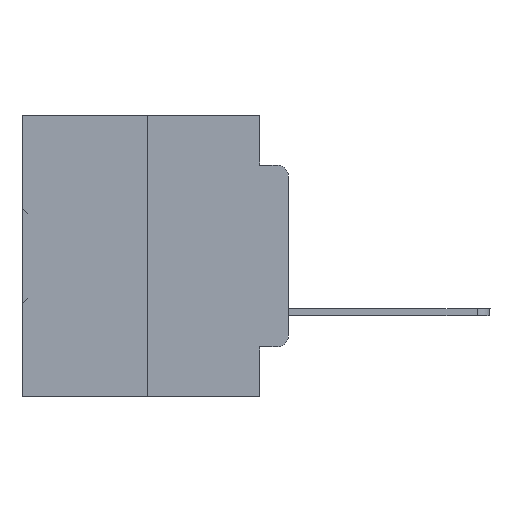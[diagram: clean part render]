
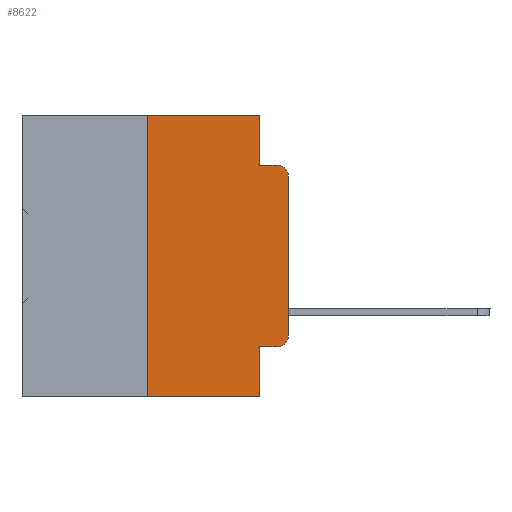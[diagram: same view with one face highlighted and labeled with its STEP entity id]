
A CAD part, left-side view. The second image highlights one B-rep face of the part: STEP entity #8622.
In plain terms, the highlighted planar face has unit normal (-1, 0, 0).
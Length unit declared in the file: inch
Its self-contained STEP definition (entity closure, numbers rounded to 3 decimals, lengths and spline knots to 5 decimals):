
#224 = EDGE_CURVE ( 'NONE', #4213, #7962, #20226, .T. ) ;
#233 = VERTEX_POINT ( 'NONE', #1468 ) ;
#249 = LINE ( 'NONE', #5409, #23473 ) ;
#731 = EDGE_CURVE ( 'NONE', #10930, #25987, #33366, .T. ) ;
#896 = FACE_OUTER_BOUND ( 'NONE', #17134, .T. ) ;
#961 = VECTOR ( 'NONE', #31922, 39.37008 ) ;
#1468 = CARTESIAN_POINT ( 'NONE',  ( 0., 0.051, -0.5 ) ) ;
#1602 = ORIENTED_EDGE ( 'NONE', *, *, #17454, .F. ) ;
#1622 = VECTOR ( 'NONE', #21729, 39.37008 ) ;
#2159 = VECTOR ( 'NONE', #25182, 39.37008 ) ;
#2207 = DIRECTION ( 'NONE',  ( 0., 0., 1. ) ) ;
#2349 = CIRCLE ( 'NONE', #22910, 0.02 ) ;
#2674 = VERTEX_POINT ( 'NONE', #13286 ) ;
#3459 = EDGE_CURVE ( 'NONE', #10445, #30776, #27428, .T. ) ;
#4138 = DIRECTION ( 'NONE',  ( 0., -1., 0. ) ) ;
#4213 = VERTEX_POINT ( 'NONE', #33942 ) ;
#4405 = ORIENTED_EDGE ( 'NONE', *, *, #32425, .T. ) ;
#4594 = CARTESIAN_POINT ( 'NONE',  ( 0., 0.473, 0. ) ) ;
#5305 = CARTESIAN_POINT ( 'NONE',  ( 0., 0.051, 0. ) ) ;
#5409 = CARTESIAN_POINT ( 'NONE',  ( 0., 0.25, 0. ) ) ;
#5776 = ORIENTED_EDGE ( 'NONE', *, *, #18271, .T. ) ;
#5810 = LINE ( 'NONE', #21061, #961 ) ;
#6533 = CARTESIAN_POINT ( 'NONE',  ( 0., 0., -0.3915 ) ) ;
#7246 = VECTOR ( 'NONE', #4138, 39.37008 ) ;
#7550 = LINE ( 'NONE', #11608, #2159 ) ;
#7962 = VERTEX_POINT ( 'NONE', #21641 ) ;
#8103 = AXIS2_PLACEMENT_3D ( 'NONE', #21590, #18375, #10329 ) ;
#8622 = ADVANCED_FACE ( 'NONE', ( #896 ), #30852, .F. ) ;
#8939 = CARTESIAN_POINT ( 'NONE',  ( 0., 0.051, -0.0885 ) ) ;
#9610 = DIRECTION ( 'NONE',  ( 0., 0., -1. ) ) ;
#10070 = DIRECTION ( 'NONE',  ( -1., 0., 0. ) ) ;
#10104 = CARTESIAN_POINT ( 'NONE',  ( 0., 0.473, -0.5 ) ) ;
#10329 = DIRECTION ( 'NONE',  ( 0., 0., -1. ) ) ;
#10389 = EDGE_CURVE ( 'NONE', #2674, #233, #34536, .T. ) ;
#10445 = VERTEX_POINT ( 'NONE', #32212 ) ;
#10621 = ORIENTED_EDGE ( 'NONE', *, *, #3459, .F. ) ;
#10930 = VERTEX_POINT ( 'NONE', #12224 ) ;
#11608 = CARTESIAN_POINT ( 'NONE',  ( 0., 0.051, 0. ) ) ;
#11614 = VECTOR ( 'NONE', #14960, 39.37008 ) ;
#12224 = CARTESIAN_POINT ( 'NONE',  ( 0., 0.051, -0.0885 ) ) ;
#13286 = CARTESIAN_POINT ( 'NONE',  ( 0., 0.25, -0.5 ) ) ;
#13334 = EDGE_CURVE ( 'NONE', #4213, #233, #5810, .T. ) ;
#13383 = VECTOR ( 'NONE', #21005, 39.37008 ) ;
#13742 = VECTOR ( 'NONE', #17152, 39.37008 ) ;
#14780 = ORIENTED_EDGE ( 'NONE', *, *, #10389, .T. ) ;
#14960 = DIRECTION ( 'NONE',  ( 0., 0., 1. ) ) ;
#14994 = EDGE_CURVE ( 'NONE', #30776, #10930, #7550, .T. ) ;
#15250 = ORIENTED_EDGE ( 'NONE', *, *, #224, .T. ) ;
#16549 = CARTESIAN_POINT ( 'NONE',  ( 0., 0.02, -0.0885 ) ) ;
#17134 = EDGE_LOOP ( 'NONE', ( #4405, #25088, #20423, #20308, #10621, #1602, #14780, #24762, #15250, #5776 ) ) ;
#17152 = DIRECTION ( 'NONE',  ( 0., -1., 0. ) ) ;
#17341 = EDGE_CURVE ( 'NONE', #23528, #25987, #2349, .T. ) ;
#17454 = EDGE_CURVE ( 'NONE', #2674, #10445, #249, .T. ) ;
#18271 = EDGE_CURVE ( 'NONE', #7962, #27362, #34887, .T. ) ;
#18322 = LINE ( 'NONE', #32039, #11614 ) ;
#18375 = DIRECTION ( 'NONE',  ( -1., 0., 0. ) ) ;
#20226 = LINE ( 'NONE', #33923, #7246 ) ;
#20308 = ORIENTED_EDGE ( 'NONE', *, *, #14994, .F. ) ;
#20423 = ORIENTED_EDGE ( 'NONE', *, *, #731, .F. ) ;
#20683 = DIRECTION ( 'NONE',  ( 1., 0., 0. ) ) ;
#21005 = DIRECTION ( 'NONE',  ( 0., -1., 0. ) ) ;
#21061 = CARTESIAN_POINT ( 'NONE',  ( 0., 0.051, 0. ) ) ;
#21590 = CARTESIAN_POINT ( 'NONE',  ( 0., 0.02, -0.3915 ) ) ;
#21641 = CARTESIAN_POINT ( 'NONE',  ( 0., 0.02, -0.4115 ) ) ;
#21729 = DIRECTION ( 'NONE',  ( 0., -1., 0. ) ) ;
#22910 = AXIS2_PLACEMENT_3D ( 'NONE', #23476, #10070, #26325 ) ;
#23473 = VECTOR ( 'NONE', #2207, 39.37008 ) ;
#23476 = CARTESIAN_POINT ( 'NONE',  ( 0., 0.02, -0.1085 ) ) ;
#23528 = VERTEX_POINT ( 'NONE', #29504 ) ;
#24226 = CARTESIAN_POINT ( 'NONE',  ( 0., 0.473, 0. ) ) ;
#24762 = ORIENTED_EDGE ( 'NONE', *, *, #13334, .F. ) ;
#25088 = ORIENTED_EDGE ( 'NONE', *, *, #17341, .T. ) ;
#25182 = DIRECTION ( 'NONE',  ( 0., 0., -1. ) ) ;
#25987 = VERTEX_POINT ( 'NONE', #16549 ) ;
#26325 = DIRECTION ( 'NONE',  ( 0., 0., -1. ) ) ;
#27362 = VERTEX_POINT ( 'NONE', #6533 ) ;
#27428 = LINE ( 'NONE', #24226, #1622 ) ;
#29504 = CARTESIAN_POINT ( 'NONE',  ( 0., 0., -0.1085 ) ) ;
#30776 = VERTEX_POINT ( 'NONE', #5305 ) ;
#30852 = PLANE ( 'NONE',  #33763 ) ;
#31922 = DIRECTION ( 'NONE',  ( 0., 0., -1. ) ) ;
#32039 = CARTESIAN_POINT ( 'NONE',  ( 0., 0., 0. ) ) ;
#32212 = CARTESIAN_POINT ( 'NONE',  ( 0., 0.25, 0. ) ) ;
#32425 = EDGE_CURVE ( 'NONE', #27362, #23528, #18322, .T. ) ;
#33366 = LINE ( 'NONE', #8939, #13742 ) ;
#33763 = AXIS2_PLACEMENT_3D ( 'NONE', #4594, #20683, #9610 ) ;
#33923 = CARTESIAN_POINT ( 'NONE',  ( 0., 0.051, -0.4115 ) ) ;
#33942 = CARTESIAN_POINT ( 'NONE',  ( 0., 0.051, -0.4115 ) ) ;
#34536 = LINE ( 'NONE', #10104, #13383 ) ;
#34887 = CIRCLE ( 'NONE', #8103, 0.02 ) ;
